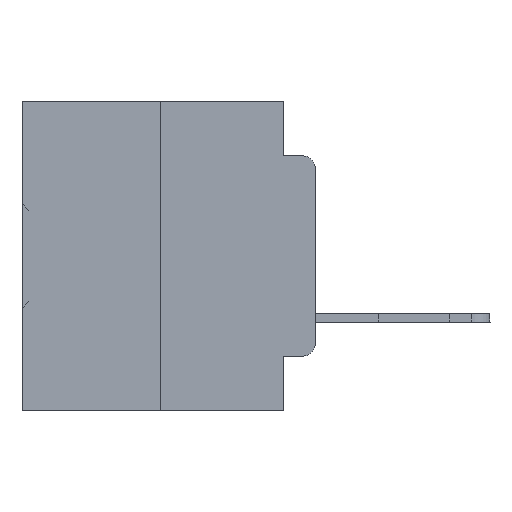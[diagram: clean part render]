
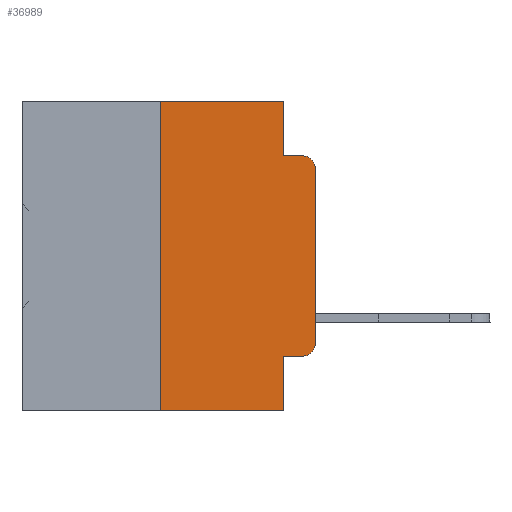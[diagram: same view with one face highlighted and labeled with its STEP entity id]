
A CAD part, left-side view. The second image highlights one B-rep face of the part: STEP entity #36989.
In plain terms, the highlighted planar face has unit normal (-1, 0, 0).
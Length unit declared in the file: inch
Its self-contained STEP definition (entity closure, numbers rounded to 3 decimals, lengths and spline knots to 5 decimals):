
#15 = AXIS2_PLACEMENT_3D ( 'NONE', #3658, #758, #8961 ) ;
#113 = LINE ( 'NONE', #20663, #29960 ) ;
#133 = VERTEX_POINT ( 'NONE', #20414 ) ;
#433 = VERTEX_POINT ( 'NONE', #31655 ) ;
#758 = DIRECTION ( 'NONE',  ( -1., 0., 0. ) ) ;
#2352 = LINE ( 'NONE', #19761, #23968 ) ;
#3062 = CARTESIAN_POINT ( 'NONE',  ( 0., 0.473, 0. ) ) ;
#3349 = ORIENTED_EDGE ( 'NONE', *, *, #14746, .T. ) ;
#3658 = CARTESIAN_POINT ( 'NONE',  ( 0., 0.02, -0.3915 ) ) ;
#3721 = DIRECTION ( 'NONE',  ( 0., 0., 1. ) ) ;
#3921 = DIRECTION ( 'NONE',  ( 0., -1., 0. ) ) ;
#5047 = CARTESIAN_POINT ( 'NONE',  ( 0., 0.02, -0.1085 ) ) ;
#5189 = LINE ( 'NONE', #3062, #27339 ) ;
#5593 = DIRECTION ( 'NONE',  ( 1., 0., 0. ) ) ;
#6751 = CARTESIAN_POINT ( 'NONE',  ( 0., 0.02, -0.4115 ) ) ;
#7900 = LINE ( 'NONE', #20793, #36397 ) ;
#8788 = EDGE_CURVE ( 'NONE', #15904, #29762, #113, .T. ) ;
#8857 = CARTESIAN_POINT ( 'NONE',  ( 0., 0.25, 0. ) ) ;
#8961 = DIRECTION ( 'NONE',  ( 0., 0., -1. ) ) ;
#9193 = VERTEX_POINT ( 'NONE', #23232 ) ;
#9483 = ORIENTED_EDGE ( 'NONE', *, *, #14957, .T. ) ;
#9727 = AXIS2_PLACEMENT_3D ( 'NONE', #5047, #19078, #33874 ) ;
#9949 = CARTESIAN_POINT ( 'NONE',  ( 0., 0., -0.3915 ) ) ;
#10845 = VERTEX_POINT ( 'NONE', #32909 ) ;
#13076 = EDGE_CURVE ( 'NONE', #13171, #133, #7900, .T. ) ;
#13171 = VERTEX_POINT ( 'NONE', #9949 ) ;
#13469 = LINE ( 'NONE', #31119, #23779 ) ;
#14567 = DIRECTION ( 'NONE',  ( 0., 0., 1. ) ) ;
#14746 = EDGE_CURVE ( 'NONE', #31401, #433, #2352, .T. ) ;
#14957 = EDGE_CURVE ( 'NONE', #133, #10845, #28105, .T. ) ;
#15385 = CIRCLE ( 'NONE', #15, 0.02 ) ;
#15768 = VERTEX_POINT ( 'NONE', #6751 ) ;
#15904 = VERTEX_POINT ( 'NONE', #18635 ) ;
#16117 = VERTEX_POINT ( 'NONE', #31680 ) ;
#17122 = DIRECTION ( 'NONE',  ( 0., 0., -1. ) ) ;
#17878 = LINE ( 'NONE', #8857, #18822 ) ;
#18270 = CARTESIAN_POINT ( 'NONE',  ( 0., 0.051, -0.0885 ) ) ;
#18635 = CARTESIAN_POINT ( 'NONE',  ( 0., 0.051, 0. ) ) ;
#18755 = EDGE_CURVE ( 'NONE', #29762, #10845, #20655, .T. ) ;
#18822 = VECTOR ( 'NONE', #14567, 39.37008 ) ;
#19078 = DIRECTION ( 'NONE',  ( -1., 0., 0. ) ) ;
#19401 = CARTESIAN_POINT ( 'NONE',  ( 0., 0.25, -0.5 ) ) ;
#19761 = CARTESIAN_POINT ( 'NONE',  ( 0., 0.473, -0.5 ) ) ;
#19794 = EDGE_CURVE ( 'NONE', #16117, #15768, #21537, .T. ) ;
#20414 = CARTESIAN_POINT ( 'NONE',  ( 0., 0., -0.1085 ) ) ;
#20655 = LINE ( 'NONE', #18270, #25223 ) ;
#20663 = CARTESIAN_POINT ( 'NONE',  ( 0., 0.051, 0. ) ) ;
#20767 = ORIENTED_EDGE ( 'NONE', *, *, #31804, .T. ) ;
#20793 = CARTESIAN_POINT ( 'NONE',  ( 0., 0., 0. ) ) ;
#21090 = ORIENTED_EDGE ( 'NONE', *, *, #18755, .F. ) ;
#21269 = CARTESIAN_POINT ( 'NONE',  ( 0., 0.051, -0.4115 ) ) ;
#21537 = LINE ( 'NONE', #21269, #23714 ) ;
#22075 = CARTESIAN_POINT ( 'NONE',  ( 0., 0.473, 0. ) ) ;
#23232 = CARTESIAN_POINT ( 'NONE',  ( 0., 0.25, 0. ) ) ;
#23527 = DIRECTION ( 'NONE',  ( 0., -1., 0. ) ) ;
#23714 = VECTOR ( 'NONE', #3921, 39.37008 ) ;
#23779 = VECTOR ( 'NONE', #28440, 39.37008 ) ;
#23968 = VECTOR ( 'NONE', #34170, 39.37008 ) ;
#24522 = EDGE_CURVE ( 'NONE', #31401, #9193, #17878, .T. ) ;
#25087 = ORIENTED_EDGE ( 'NONE', *, *, #37337, .F. ) ;
#25223 = VECTOR ( 'NONE', #32953, 39.37008 ) ;
#25534 = AXIS2_PLACEMENT_3D ( 'NONE', #22075, #5593, #17122 ) ;
#27004 = ORIENTED_EDGE ( 'NONE', *, *, #19794, .T. ) ;
#27339 = VECTOR ( 'NONE', #23527, 39.37008 ) ;
#28035 = CARTESIAN_POINT ( 'NONE',  ( 0., 0.051, -0.0885 ) ) ;
#28105 = CIRCLE ( 'NONE', #9727, 0.02 ) ;
#28440 = DIRECTION ( 'NONE',  ( 0., 0., -1. ) ) ;
#29037 = DIRECTION ( 'NONE',  ( 0., 0., -1. ) ) ;
#29148 = ORIENTED_EDGE ( 'NONE', *, *, #30265, .F. ) ;
#29762 = VERTEX_POINT ( 'NONE', #28035 ) ;
#29960 = VECTOR ( 'NONE', #29037, 39.37008 ) ;
#30265 = EDGE_CURVE ( 'NONE', #16117, #433, #13469, .T. ) ;
#31110 = EDGE_LOOP ( 'NONE', ( #33140, #9483, #21090, #31261, #25087, #37348, #3349, #29148, #27004, #20767 ) ) ;
#31119 = CARTESIAN_POINT ( 'NONE',  ( 0., 0.051, 0. ) ) ;
#31261 = ORIENTED_EDGE ( 'NONE', *, *, #8788, .F. ) ;
#31401 = VERTEX_POINT ( 'NONE', #19401 ) ;
#31469 = FACE_OUTER_BOUND ( 'NONE', #31110, .T. ) ;
#31655 = CARTESIAN_POINT ( 'NONE',  ( 0., 0.051, -0.5 ) ) ;
#31680 = CARTESIAN_POINT ( 'NONE',  ( 0., 0.051, -0.4115 ) ) ;
#31804 = EDGE_CURVE ( 'NONE', #15768, #13171, #15385, .T. ) ;
#32034 = PLANE ( 'NONE',  #25534 ) ;
#32909 = CARTESIAN_POINT ( 'NONE',  ( 0., 0.02, -0.0885 ) ) ;
#32953 = DIRECTION ( 'NONE',  ( 0., -1., 0. ) ) ;
#33140 = ORIENTED_EDGE ( 'NONE', *, *, #13076, .T. ) ;
#33874 = DIRECTION ( 'NONE',  ( 0., 0., -1. ) ) ;
#34170 = DIRECTION ( 'NONE',  ( 0., -1., 0. ) ) ;
#36397 = VECTOR ( 'NONE', #3721, 39.37008 ) ;
#36989 = ADVANCED_FACE ( 'NONE', ( #31469 ), #32034, .F. ) ;
#37337 = EDGE_CURVE ( 'NONE', #9193, #15904, #5189, .T. ) ;
#37348 = ORIENTED_EDGE ( 'NONE', *, *, #24522, .F. ) ;
